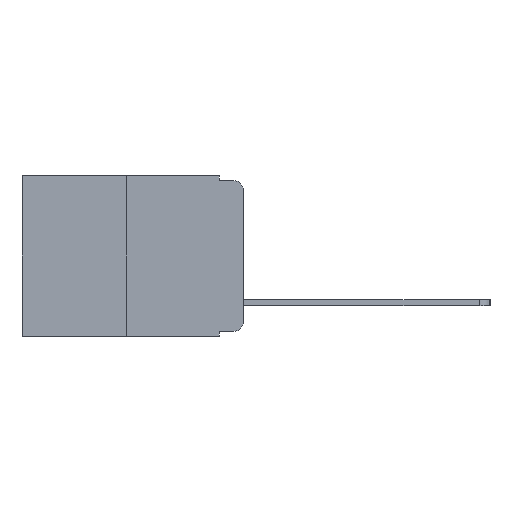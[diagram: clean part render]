
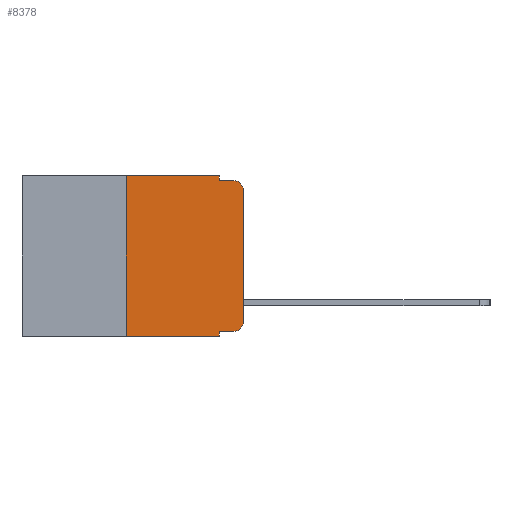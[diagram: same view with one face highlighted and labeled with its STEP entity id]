
A CAD part, left-side view. The second image highlights one B-rep face of the part: STEP entity #8378.
In plain terms, the highlighted planar face has unit normal (-1, 0, 0).
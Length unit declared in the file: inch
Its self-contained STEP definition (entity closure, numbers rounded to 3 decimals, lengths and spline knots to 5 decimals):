
#33 = CARTESIAN_POINT ( 'NONE',  ( 0., 0.25, 0. ) ) ;
#129 = VECTOR ( 'NONE', #17034, 39.37008 ) ;
#163 = CARTESIAN_POINT ( 'NONE',  ( 0., 0., -0.313 ) ) ;
#537 = VECTOR ( 'NONE', #17862, 39.37008 ) ;
#634 = CARTESIAN_POINT ( 'NONE',  ( 0., 0.473, 0. ) ) ;
#977 = ORIENTED_EDGE ( 'NONE', *, *, #8831, .T. ) ;
#1175 = LINE ( 'NONE', #33, #9068 ) ;
#1372 = CIRCLE ( 'NONE', #17268, 0.02 ) ;
#1438 = ORIENTED_EDGE ( 'NONE', *, *, #17596, .F. ) ;
#2008 = EDGE_CURVE ( 'NONE', #3649, #14666, #14365, .T. ) ;
#2169 = DIRECTION ( 'NONE',  ( 0., -1., 0. ) ) ;
#2679 = LINE ( 'NONE', #12594, #10420 ) ;
#2793 = DIRECTION ( 'NONE',  ( 0., -1., 0. ) ) ;
#2841 = VECTOR ( 'NONE', #2169, 39.37008 ) ;
#2927 = EDGE_CURVE ( 'NONE', #14666, #7979, #5641, .T. ) ;
#2976 = VERTEX_POINT ( 'NONE', #2980 ) ;
#2980 = CARTESIAN_POINT ( 'NONE',  ( 0., 0.25, -0.343 ) ) ;
#3349 = CARTESIAN_POINT ( 'NONE',  ( 0., 0.02, -0.333 ) ) ;
#3649 = VERTEX_POINT ( 'NONE', #14608 ) ;
#3726 = VERTEX_POINT ( 'NONE', #163 ) ;
#3948 = EDGE_CURVE ( 'NONE', #7979, #13989, #6723, .T. ) ;
#3974 = DIRECTION ( 'NONE',  ( -1., 0., 0. ) ) ;
#4074 = PLANE ( 'NONE',  #9822 ) ;
#4143 = VECTOR ( 'NONE', #2793, 39.37008 ) ;
#4629 = LINE ( 'NONE', #10865, #537 ) ;
#4938 = EDGE_CURVE ( 'NONE', #16621, #13989, #8723, .T. ) ;
#5192 = EDGE_CURVE ( 'NONE', #2976, #16049, #12211, .T. ) ;
#5498 = VERTEX_POINT ( 'NONE', #10727 ) ;
#5575 = DIRECTION ( 'NONE',  ( 1., 0., 0. ) ) ;
#5641 = LINE ( 'NONE', #15737, #129 ) ;
#5793 = ORIENTED_EDGE ( 'NONE', *, *, #2927, .F. ) ;
#6708 = DIRECTION ( 'NONE',  ( 0., -1., 0. ) ) ;
#6723 = LINE ( 'NONE', #17928, #10495 ) ;
#7326 = VECTOR ( 'NONE', #12330, 39.37008 ) ;
#7979 = VERTEX_POINT ( 'NONE', #8983 ) ;
#8076 = VERTEX_POINT ( 'NONE', #3349 ) ;
#8184 = DIRECTION ( 'NONE',  ( -1., 0., 0. ) ) ;
#8378 = ADVANCED_FACE ( 'NONE', ( #8683 ), #4074, .F. ) ;
#8683 = FACE_OUTER_BOUND ( 'NONE', #16558, .T. ) ;
#8723 = CIRCLE ( 'NONE', #11858, 0.02 ) ;
#8831 = EDGE_CURVE ( 'NONE', #3726, #16621, #11074, .T. ) ;
#8983 = CARTESIAN_POINT ( 'NONE',  ( 0., 0.051, -0.01 ) ) ;
#9068 = VECTOR ( 'NONE', #14612, 39.37008 ) ;
#9822 = AXIS2_PLACEMENT_3D ( 'NONE', #14110, #5575, #15522 ) ;
#9851 = CARTESIAN_POINT ( 'NONE',  ( 0., 0.02, -0.01 ) ) ;
#10420 = VECTOR ( 'NONE', #13961, 39.37008 ) ;
#10495 = VECTOR ( 'NONE', #6708, 39.37008 ) ;
#10727 = CARTESIAN_POINT ( 'NONE',  ( 0., 0.051, -0.333 ) ) ;
#10865 = CARTESIAN_POINT ( 'NONE',  ( 0., 0.051, -0.333 ) ) ;
#11074 = LINE ( 'NONE', #17794, #7326 ) ;
#11205 = ORIENTED_EDGE ( 'NONE', *, *, #18529, .F. ) ;
#11419 = CARTESIAN_POINT ( 'NONE',  ( 0., 0.051, 0. ) ) ;
#11469 = CARTESIAN_POINT ( 'NONE',  ( 0., 0.473, -0.343 ) ) ;
#11858 = AXIS2_PLACEMENT_3D ( 'NONE', #16577, #8184, #17926 ) ;
#12091 = CARTESIAN_POINT ( 'NONE',  ( 0., 0., -0.03 ) ) ;
#12198 = ORIENTED_EDGE ( 'NONE', *, *, #13916, .T. ) ;
#12211 = LINE ( 'NONE', #11469, #4143 ) ;
#12330 = DIRECTION ( 'NONE',  ( 0., 0., 1. ) ) ;
#12571 = CARTESIAN_POINT ( 'NONE',  ( 0., 0.02, -0.313 ) ) ;
#12594 = CARTESIAN_POINT ( 'NONE',  ( 0., 0.051, 0. ) ) ;
#12706 = ORIENTED_EDGE ( 'NONE', *, *, #4938, .T. ) ;
#13105 = ORIENTED_EDGE ( 'NONE', *, *, #16704, .T. ) ;
#13810 = ORIENTED_EDGE ( 'NONE', *, *, #5192, .T. ) ;
#13916 = EDGE_CURVE ( 'NONE', #8076, #3726, #1372, .T. ) ;
#13961 = DIRECTION ( 'NONE',  ( 0., 0., -1. ) ) ;
#13989 = VERTEX_POINT ( 'NONE', #9851 ) ;
#14007 = DIRECTION ( 'NONE',  ( 0., 0., -1. ) ) ;
#14110 = CARTESIAN_POINT ( 'NONE',  ( 0., 0.473, 0. ) ) ;
#14365 = LINE ( 'NONE', #634, #2841 ) ;
#14608 = CARTESIAN_POINT ( 'NONE',  ( 0., 0.25, 0. ) ) ;
#14612 = DIRECTION ( 'NONE',  ( 0., 0., 1. ) ) ;
#14666 = VERTEX_POINT ( 'NONE', #11419 ) ;
#14738 = CARTESIAN_POINT ( 'NONE',  ( 0., 0.051, -0.343 ) ) ;
#14934 = ORIENTED_EDGE ( 'NONE', *, *, #3948, .F. ) ;
#15522 = DIRECTION ( 'NONE',  ( 0., 0., -1. ) ) ;
#15737 = CARTESIAN_POINT ( 'NONE',  ( 0., 0.051, 0. ) ) ;
#16049 = VERTEX_POINT ( 'NONE', #14738 ) ;
#16137 = ORIENTED_EDGE ( 'NONE', *, *, #2008, .F. ) ;
#16558 = EDGE_LOOP ( 'NONE', ( #977, #12706, #14934, #5793, #16137, #11205, #13810, #1438, #13105, #12198 ) ) ;
#16577 = CARTESIAN_POINT ( 'NONE',  ( 0., 0.02, -0.03 ) ) ;
#16621 = VERTEX_POINT ( 'NONE', #12091 ) ;
#16704 = EDGE_CURVE ( 'NONE', #5498, #8076, #4629, .T. ) ;
#17034 = DIRECTION ( 'NONE',  ( 0., 0., -1. ) ) ;
#17268 = AXIS2_PLACEMENT_3D ( 'NONE', #12571, #3974, #14007 ) ;
#17596 = EDGE_CURVE ( 'NONE', #5498, #16049, #2679, .T. ) ;
#17794 = CARTESIAN_POINT ( 'NONE',  ( 0., 0., 0. ) ) ;
#17862 = DIRECTION ( 'NONE',  ( 0., -1., 0. ) ) ;
#17926 = DIRECTION ( 'NONE',  ( 0., 0., -1. ) ) ;
#17928 = CARTESIAN_POINT ( 'NONE',  ( 0., 0.051, -0.01 ) ) ;
#18529 = EDGE_CURVE ( 'NONE', #2976, #3649, #1175, .T. ) ;
